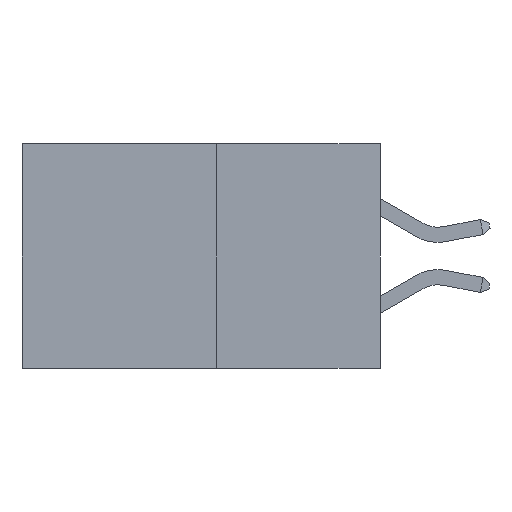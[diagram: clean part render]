
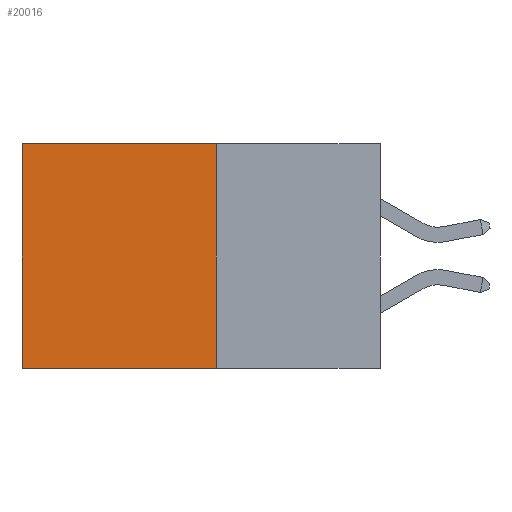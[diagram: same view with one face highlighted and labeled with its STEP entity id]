
A CAD part, left-side view. The second image highlights one B-rep face of the part: STEP entity #20016.
In plain terms, the highlighted planar face has unit normal (-1, 0, 0).
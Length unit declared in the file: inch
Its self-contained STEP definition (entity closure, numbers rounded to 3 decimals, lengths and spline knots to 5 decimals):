
#894 = ORIENTED_EDGE ( 'NONE', *, *, #13248, .F. ) ;
#977 = CARTESIAN_POINT ( 'NONE',  ( 0.277, 0.27, -0.37 ) ) ;
#2614 = CARTESIAN_POINT ( 'NONE',  ( 0.277, 0.27, -0.37 ) ) ;
#4241 = VERTEX_POINT ( 'NONE', #977 ) ;
#4601 = EDGE_CURVE ( 'NONE', #20046, #15649, #10723, .T. ) ;
#4742 = ORIENTED_EDGE ( 'NONE', *, *, #20652, .T. ) ;
#4747 = VECTOR ( 'NONE', #13315, 39.37008 ) ;
#5623 = VECTOR ( 'NONE', #23602, 39.37008 ) ;
#6340 = CARTESIAN_POINT ( 'NONE',  ( 0.277, 0.59, -0.37 ) ) ;
#6408 = LINE ( 'NONE', #6340, #5623 ) ;
#6550 = LINE ( 'NONE', #2614, #19725 ) ;
#7772 = CARTESIAN_POINT ( 'NONE',  ( 0.277, 0.59, 0. ) ) ;
#8008 = VERTEX_POINT ( 'NONE', #15394 ) ;
#10360 = FACE_OUTER_BOUND ( 'NONE', #21754, .T. ) ;
#10723 = LINE ( 'NONE', #15387, #17263 ) ;
#10843 = CARTESIAN_POINT ( 'NONE',  ( 0.277, 0.27, -0.37 ) ) ;
#11389 = LINE ( 'NONE', #10843, #4747 ) ;
#12587 = CARTESIAN_POINT ( 'NONE',  ( 0.277, 0.27, -0.37 ) ) ;
#12699 = CARTESIAN_POINT ( 'NONE',  ( 0.277, 0.27, 0. ) ) ;
#12948 = AXIS2_PLACEMENT_3D ( 'NONE', #12587, #29703, #15053 ) ;
#13248 = EDGE_CURVE ( 'NONE', #20046, #4241, #11389, .T. ) ;
#13315 = DIRECTION ( 'NONE',  ( 0., 0., -1. ) ) ;
#15001 = DIRECTION ( 'NONE',  ( 0., 1., 0. ) ) ;
#15053 = DIRECTION ( 'NONE',  ( 0., 0., -1. ) ) ;
#15387 = CARTESIAN_POINT ( 'NONE',  ( 0.277, 0.27, 0. ) ) ;
#15394 = CARTESIAN_POINT ( 'NONE',  ( 0.277, 0.59, -0.37 ) ) ;
#15649 = VERTEX_POINT ( 'NONE', #7772 ) ;
#16310 = EDGE_CURVE ( 'NONE', #4241, #8008, #6550, .T. ) ;
#17263 = VECTOR ( 'NONE', #15001, 39.37008 ) ;
#17431 = PLANE ( 'NONE',  #12948 ) ;
#19725 = VECTOR ( 'NONE', #19962, 39.37008 ) ;
#19962 = DIRECTION ( 'NONE',  ( 0., 1., 0. ) ) ;
#20016 = ADVANCED_FACE ( 'NONE', ( #10360 ), #17431, .F. ) ;
#20046 = VERTEX_POINT ( 'NONE', #12699 ) ;
#20652 = EDGE_CURVE ( 'NONE', #15649, #8008, #6408, .T. ) ;
#20826 = ORIENTED_EDGE ( 'NONE', *, *, #16310, .F. ) ;
#21754 = EDGE_LOOP ( 'NONE', ( #4742, #20826, #894, #27276 ) ) ;
#23602 = DIRECTION ( 'NONE',  ( 0., 0., -1. ) ) ;
#27276 = ORIENTED_EDGE ( 'NONE', *, *, #4601, .T. ) ;
#29703 = DIRECTION ( 'NONE',  ( 1., 0., 0. ) ) ;
